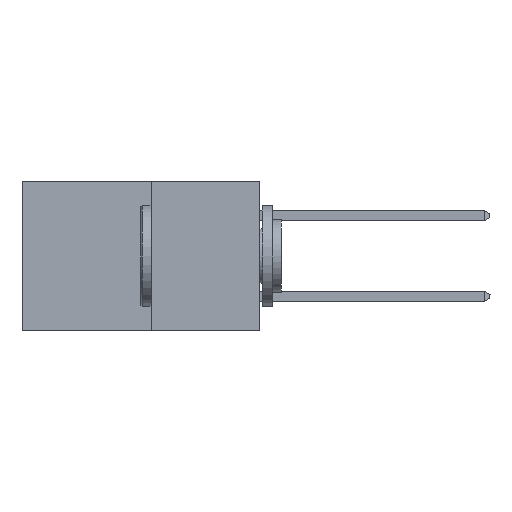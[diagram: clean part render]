
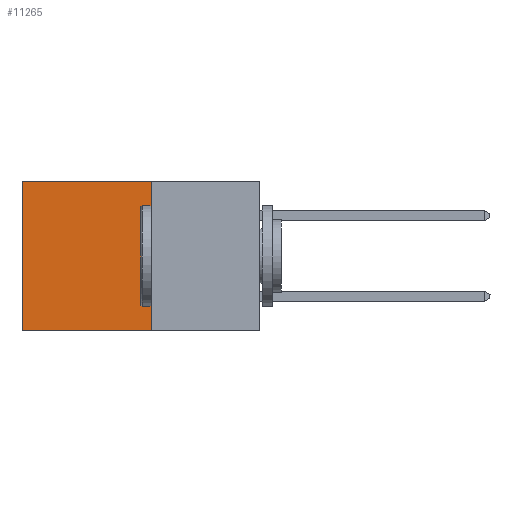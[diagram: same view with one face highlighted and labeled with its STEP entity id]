
A CAD part, left-side view. The second image highlights one B-rep face of the part: STEP entity #11265.
In plain terms, the highlighted planar face has unit normal (-1, 0, 0).
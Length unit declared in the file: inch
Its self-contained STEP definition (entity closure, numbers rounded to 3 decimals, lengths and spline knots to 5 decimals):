
#436 = ORIENTED_EDGE ( 'NONE', *, *, #12492, .T. ) ;
#556 = VERTEX_POINT ( 'NONE', #3693 ) ;
#691 = CARTESIAN_POINT ( 'NONE',  ( 0.277, 0.27, -0.37 ) ) ;
#1456 = DIRECTION ( 'NONE',  ( 1., 0., 0. ) ) ;
#2050 = VERTEX_POINT ( 'NONE', #8283 ) ;
#3262 = VERTEX_POINT ( 'NONE', #16152 ) ;
#3693 = CARTESIAN_POINT ( 'NONE',  ( 0.277, 0.59, 0. ) ) ;
#4909 = CARTESIAN_POINT ( 'NONE',  ( 0.277, 0.27, -0.37 ) ) ;
#5463 = ORIENTED_EDGE ( 'NONE', *, *, #6436, .F. ) ;
#6436 = EDGE_CURVE ( 'NONE', #3262, #24694, #18706, .T. ) ;
#7185 = DIRECTION ( 'NONE',  ( 0., 0., -1. ) ) ;
#7317 = PLANE ( 'NONE',  #20929 ) ;
#8283 = CARTESIAN_POINT ( 'NONE',  ( 0.277, 0.59, -0.37 ) ) ;
#10296 = ORIENTED_EDGE ( 'NONE', *, *, #15816, .F. ) ;
#11265 = ADVANCED_FACE ( 'NONE', ( #20472 ), #7317, .F. ) ;
#11307 = CARTESIAN_POINT ( 'NONE',  ( 0.277, 0.27, -0.37 ) ) ;
#12110 = LINE ( 'NONE', #691, #22046 ) ;
#12492 = EDGE_CURVE ( 'NONE', #556, #2050, #18258, .T. ) ;
#12708 = DIRECTION ( 'NONE',  ( 0., 1., 0. ) ) ;
#15317 = DIRECTION ( 'NONE',  ( 0., 0., -1. ) ) ;
#15816 = EDGE_CURVE ( 'NONE', #24694, #2050, #12110, .T. ) ;
#16085 = EDGE_LOOP ( 'NONE', ( #436, #10296, #5463, #21720 ) ) ;
#16152 = CARTESIAN_POINT ( 'NONE',  ( 0.277, 0.27, 0. ) ) ;
#17636 = VECTOR ( 'NONE', #7185, 39.37008 ) ;
#18258 = LINE ( 'NONE', #24893, #17636 ) ;
#18289 = CARTESIAN_POINT ( 'NONE',  ( 0.277, 0.27, -0.37 ) ) ;
#18706 = LINE ( 'NONE', #4909, #23905 ) ;
#20347 = DIRECTION ( 'NONE',  ( 0., 1., 0. ) ) ;
#20472 = FACE_OUTER_BOUND ( 'NONE', #16085, .T. ) ;
#20929 = AXIS2_PLACEMENT_3D ( 'NONE', #11307, #1456, #15317 ) ;
#21720 = ORIENTED_EDGE ( 'NONE', *, *, #25262, .T. ) ;
#22046 = VECTOR ( 'NONE', #20347, 39.37008 ) ;
#22975 = LINE ( 'NONE', #24531, #24184 ) ;
#23905 = VECTOR ( 'NONE', #24673, 39.37008 ) ;
#24184 = VECTOR ( 'NONE', #12708, 39.37008 ) ;
#24531 = CARTESIAN_POINT ( 'NONE',  ( 0.277, 0.27, 0. ) ) ;
#24673 = DIRECTION ( 'NONE',  ( 0., 0., -1. ) ) ;
#24694 = VERTEX_POINT ( 'NONE', #18289 ) ;
#24893 = CARTESIAN_POINT ( 'NONE',  ( 0.277, 0.59, -0.37 ) ) ;
#25262 = EDGE_CURVE ( 'NONE', #3262, #556, #22975, .T. ) ;
